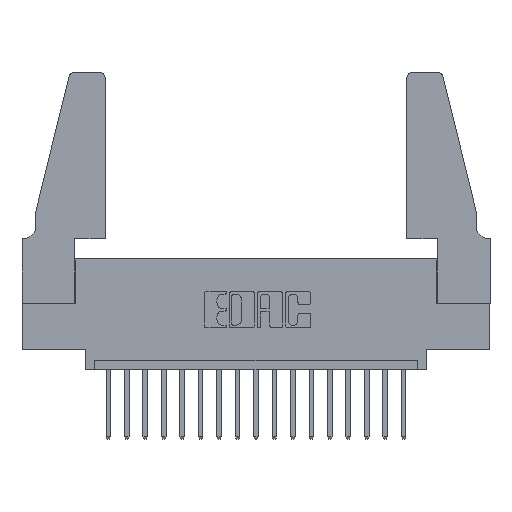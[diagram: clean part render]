
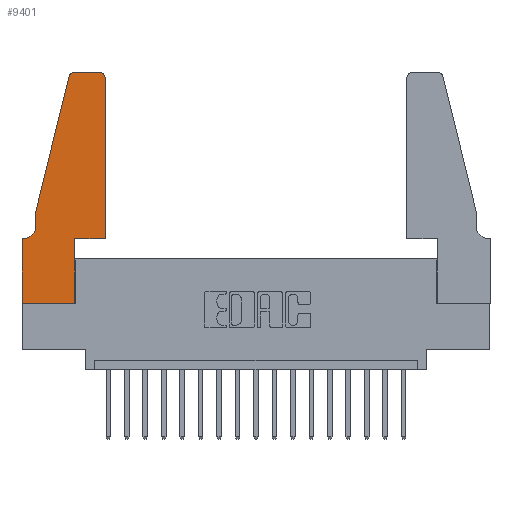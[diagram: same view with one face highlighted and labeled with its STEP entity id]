
A CAD part, top view. The second image highlights one B-rep face of the part: STEP entity #9401.
In plain terms, the highlighted planar face has unit normal (0, 0, 1).
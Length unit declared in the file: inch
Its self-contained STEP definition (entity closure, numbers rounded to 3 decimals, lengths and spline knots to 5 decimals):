
#554 = AXIS2_PLACEMENT_3D ( 'NONE', #13388, #564, #13509 ) ;
#564 = DIRECTION ( 'NONE',  ( 0., 0., 1. ) ) ;
#752 = CARTESIAN_POINT ( 'NONE',  ( 0.4505, 0.35, 0.37 ) ) ;
#1019 = DIRECTION ( 'NONE',  ( 0., 1., 0. ) ) ;
#1248 = EDGE_CURVE ( 'NONE', #12913, #16269, #18447, .T. ) ;
#1608 = CARTESIAN_POINT ( 'NONE',  ( 0., 0., 0.37 ) ) ;
#1957 = CIRCLE ( 'NONE', #3459, 0.03 ) ;
#2298 = EDGE_CURVE ( 'NONE', #11254, #15125, #16217, .T. ) ;
#2431 = VECTOR ( 'NONE', #10931, 39.37008 ) ;
#2981 = DIRECTION ( 'NONE',  ( 0., 0., 1. ) ) ;
#3146 = ORIENTED_EDGE ( 'NONE', *, *, #14211, .T. ) ;
#3149 = ORIENTED_EDGE ( 'NONE', *, *, #12692, .T. ) ;
#3350 = AXIS2_PLACEMENT_3D ( 'NONE', #4952, #2981, #10191 ) ;
#3387 = LINE ( 'NONE', #15194, #18097 ) ;
#3445 = ORIENTED_EDGE ( 'NONE', *, *, #6006, .T. ) ;
#3459 = AXIS2_PLACEMENT_3D ( 'NONE', #10298, #10110, #11653 ) ;
#3602 = VERTEX_POINT ( 'NONE', #9102 ) ;
#3807 = LINE ( 'NONE', #13014, #10732 ) ;
#4408 = ORIENTED_EDGE ( 'NONE', *, *, #12463, .T. ) ;
#4478 = DIRECTION ( 'NONE',  ( -1., 0., 0. ) ) ;
#4759 = DIRECTION ( 'NONE',  ( 0., -1., 0. ) ) ;
#4952 = CARTESIAN_POINT ( 'NONE',  ( 0., 0.35, 0.37 ) ) ;
#5622 = EDGE_CURVE ( 'NONE', #16725, #16905, #17642, .T. ) ;
#5946 = FACE_OUTER_BOUND ( 'NONE', #11138, .T. ) ;
#6006 = EDGE_CURVE ( 'NONE', #11634, #16609, #17843, .T. ) ;
#6023 = CARTESIAN_POINT ( 'NONE',  ( 0.2865, 0., 0.37 ) ) ;
#6524 = VECTOR ( 'NONE', #4759, 39.37008 ) ;
#6850 = CARTESIAN_POINT ( 'NONE',  ( 0.0755, 0.35, 0.37 ) ) ;
#7205 = CARTESIAN_POINT ( 'NONE',  ( 0., 0., 0.37 ) ) ;
#7268 = CARTESIAN_POINT ( 'NONE',  ( 0.4205, 1.25, 0.37 ) ) ;
#7310 = DIRECTION ( 'NONE',  ( 1., 0., 0. ) ) ;
#7558 = EDGE_CURVE ( 'NONE', #8493, #11254, #1957, .T. ) ;
#7660 = CARTESIAN_POINT ( 'NONE',  ( 0.25487, 1.22718, 0.37 ) ) ;
#7856 = LINE ( 'NONE', #16706, #15848 ) ;
#7870 = DIRECTION ( 'NONE',  ( 0., 1., 0. ) ) ;
#8182 = VECTOR ( 'NONE', #16873, 39.37008 ) ;
#8247 = VECTOR ( 'NONE', #7310, 39.37008 ) ;
#8307 = ORIENTED_EDGE ( 'NONE', *, *, #17025, .T. ) ;
#8458 = ORIENTED_EDGE ( 'NONE', *, *, #17395, .T. ) ;
#8493 = VERTEX_POINT ( 'NONE', #12694 ) ;
#8706 = DIRECTION ( 'NONE',  ( -1., 0., 0. ) ) ;
#8750 = LINE ( 'NONE', #16034, #6524 ) ;
#9102 = CARTESIAN_POINT ( 'NONE',  ( 0.0055, 0.35, 0.37 ) ) ;
#9401 = ADVANCED_FACE ( 'NONE', ( #5946 ), #17711, .T. ) ;
#9854 = EDGE_CURVE ( 'NONE', #3602, #15313, #14652, .T. ) ;
#10077 = DIRECTION ( 'NONE',  ( 0., -1., 0. ) ) ;
#10084 = VERTEX_POINT ( 'NONE', #10378 ) ;
#10110 = DIRECTION ( 'NONE',  ( 0., 0., 1. ) ) ;
#10178 = ORIENTED_EDGE ( 'NONE', *, *, #9854, .T. ) ;
#10191 = DIRECTION ( 'NONE',  ( 1., 0., 0. ) ) ;
#10298 = CARTESIAN_POINT ( 'NONE',  ( 0.284, 1.22, 0.37 ) ) ;
#10378 = CARTESIAN_POINT ( 'NONE',  ( 0.0755, 0.42, 0.37 ) ) ;
#10657 = CARTESIAN_POINT ( 'NONE',  ( 0.4505, 1.22, 0.37 ) ) ;
#10732 = VECTOR ( 'NONE', #4478, 39.37008 ) ;
#10931 = DIRECTION ( 'NONE',  ( 1., 0., 0. ) ) ;
#11138 = EDGE_LOOP ( 'NONE', ( #4408, #14626, #11188, #8307, #3146, #10178, #3149, #14401, #16498, #3445, #8458, #13906 ) ) ;
#11188 = ORIENTED_EDGE ( 'NONE', *, *, #2298, .T. ) ;
#11254 = VERTEX_POINT ( 'NONE', #7660 ) ;
#11634 = VERTEX_POINT ( 'NONE', #13087 ) ;
#11653 = DIRECTION ( 'NONE',  ( 1., 0., 0. ) ) ;
#11736 = EDGE_CURVE ( 'NONE', #16269, #11634, #3387, .T. ) ;
#12463 = EDGE_CURVE ( 'NONE', #16905, #8493, #3807, .T. ) ;
#12692 = EDGE_CURVE ( 'NONE', #15313, #12913, #16030, .T. ) ;
#12694 = CARTESIAN_POINT ( 'NONE',  ( 0.284, 1.25, 0.37 ) ) ;
#12779 = CARTESIAN_POINT ( 'NONE',  ( 0., 0., 0.37 ) ) ;
#12913 = VERTEX_POINT ( 'NONE', #1608 ) ;
#13014 = CARTESIAN_POINT ( 'NONE',  ( 0.2605, 1.25, 0.37 ) ) ;
#13087 = CARTESIAN_POINT ( 'NONE',  ( 0.2865, 0.35, 0.37 ) ) ;
#13350 = CARTESIAN_POINT ( 'NONE',  ( 0.0755, 0.5, 0.37 ) ) ;
#13388 = CARTESIAN_POINT ( 'NONE',  ( 0.4205, 1.22, 0.37 ) ) ;
#13509 = DIRECTION ( 'NONE',  ( 1., 0., 0. ) ) ;
#13906 = ORIENTED_EDGE ( 'NONE', *, *, #5622, .T. ) ;
#14211 = EDGE_CURVE ( 'NONE', #10084, #3602, #15721, .T. ) ;
#14262 = CARTESIAN_POINT ( 'NONE',  ( 0.0055, 0.42, 0.37 ) ) ;
#14401 = ORIENTED_EDGE ( 'NONE', *, *, #1248, .T. ) ;
#14626 = ORIENTED_EDGE ( 'NONE', *, *, #7558, .T. ) ;
#14652 = LINE ( 'NONE', #6850, #8182 ) ;
#15125 = VERTEX_POINT ( 'NONE', #13350 ) ;
#15194 = CARTESIAN_POINT ( 'NONE',  ( 0.2865, 0.35, 0.37 ) ) ;
#15213 = AXIS2_PLACEMENT_3D ( 'NONE', #14262, #15661, #8706 ) ;
#15313 = VERTEX_POINT ( 'NONE', #16929 ) ;
#15661 = DIRECTION ( 'NONE',  ( 0., 0., -1. ) ) ;
#15721 = CIRCLE ( 'NONE', #15213, 0.07 ) ;
#15846 = DIRECTION ( 'NONE',  ( -0.239, -0.971, 0. ) ) ;
#15848 = VECTOR ( 'NONE', #1019, 39.37008 ) ;
#15990 = VECTOR ( 'NONE', #15846, 39.37008 ) ;
#16030 = LINE ( 'NONE', #7205, #17359 ) ;
#16034 = CARTESIAN_POINT ( 'NONE',  ( 0.0755, 0.5, 0.37 ) ) ;
#16217 = LINE ( 'NONE', #17358, #15990 ) ;
#16269 = VERTEX_POINT ( 'NONE', #6023 ) ;
#16498 = ORIENTED_EDGE ( 'NONE', *, *, #11736, .T. ) ;
#16609 = VERTEX_POINT ( 'NONE', #18288 ) ;
#16706 = CARTESIAN_POINT ( 'NONE',  ( 0.4505, 0.35, 0.37 ) ) ;
#16725 = VERTEX_POINT ( 'NONE', #10657 ) ;
#16873 = DIRECTION ( 'NONE',  ( -1., 0., 0. ) ) ;
#16905 = VERTEX_POINT ( 'NONE', #7268 ) ;
#16929 = CARTESIAN_POINT ( 'NONE',  ( 0., 0.35, 0.37 ) ) ;
#17025 = EDGE_CURVE ( 'NONE', #15125, #10084, #8750, .T. ) ;
#17358 = CARTESIAN_POINT ( 'NONE',  ( 0.0755, 0.5, 0.37 ) ) ;
#17359 = VECTOR ( 'NONE', #10077, 39.37008 ) ;
#17395 = EDGE_CURVE ( 'NONE', #16609, #16725, #7856, .T. ) ;
#17642 = CIRCLE ( 'NONE', #554, 0.03 ) ;
#17711 = PLANE ( 'NONE',  #3350 ) ;
#17843 = LINE ( 'NONE', #752, #2431 ) ;
#18097 = VECTOR ( 'NONE', #7870, 39.37008 ) ;
#18288 = CARTESIAN_POINT ( 'NONE',  ( 0.4505, 0.35, 0.37 ) ) ;
#18447 = LINE ( 'NONE', #12779, #8247 ) ;
